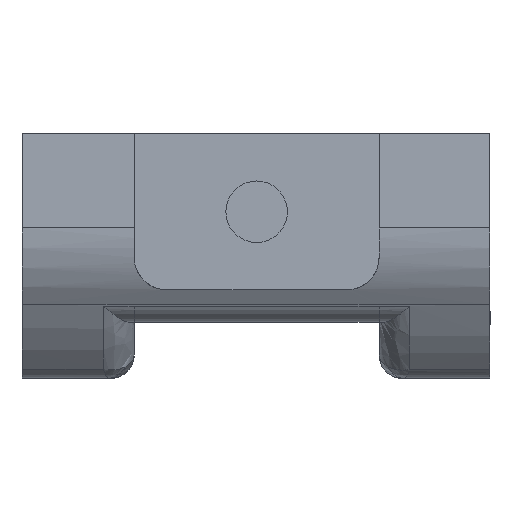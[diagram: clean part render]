
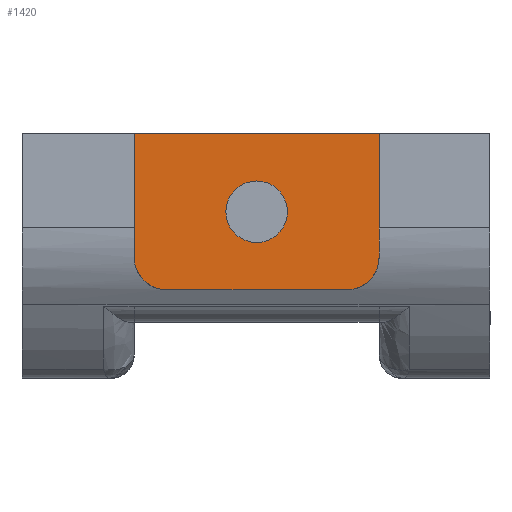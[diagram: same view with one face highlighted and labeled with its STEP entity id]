
A CAD part, front view. The second image highlights one B-rep face of the part: STEP entity #1420.
In plain terms, the highlighted planar face has unit normal (0, -1, 0).
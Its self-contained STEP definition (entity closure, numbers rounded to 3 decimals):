
#122 = AXIS2_PLACEMENT_3D ( 'NONE', #3254, #1624, #817 ) ;
#136 = VERTEX_POINT ( 'NONE', #1175 ) ;
#145 = ORIENTED_EDGE ( 'NONE', *, *, #2261, .F. ) ;
#321 = EDGE_CURVE ( 'NONE', #1790, #3347, #2233, .T. ) ;
#439 = AXIS2_PLACEMENT_3D ( 'NONE', #2309, #3396, #2859 ) ;
#485 = CARTESIAN_POINT ( 'NONE',  ( 0., 3.175, -5.31 ) ) ;
#489 = EDGE_CURVE ( 'NONE', #3307, #1974, #1639, .T. ) ;
#499 = CIRCLE ( 'NONE', #439, 1.5 ) ;
#536 = CARTESIAN_POINT ( 'NONE',  ( -4.381, 3.175, -6.032 ) ) ;
#575 = ORIENTED_EDGE ( 'NONE', *, *, #489, .T. ) ;
#640 = LINE ( 'NONE', #1937, #2943 ) ;
#683 = FACE_BOUND ( 'NONE', #936, .T. ) ;
#817 = DIRECTION ( 'NONE',  ( 0., 0., -1. ) ) ;
#936 = EDGE_LOOP ( 'NONE', ( #2551, #145 ) ) ;
#1020 = CARTESIAN_POINT ( 'NONE',  ( 5.969, 3.175, 0. ) ) ;
#1175 = CARTESIAN_POINT ( 'NONE',  ( -5.969, 3.175, 0. ) ) ;
#1206 = CIRCLE ( 'NONE', #122, 1.5 ) ;
#1323 = VERTEX_POINT ( 'NONE', #3058 ) ;
#1327 = DIRECTION ( 'NONE',  ( 1., 0., 0. ) ) ;
#1420 = ADVANCED_FACE ( 'NONE', ( #683, #3159 ), #2079, .T. ) ;
#1427 = VECTOR ( 'NONE', #2597, 1000. ) ;
#1436 = VECTOR ( 'NONE', #2365, 1000. ) ;
#1464 = CARTESIAN_POINT ( 'NONE',  ( 4.381, 3.175, -6.032 ) ) ;
#1465 = AXIS2_PLACEMENT_3D ( 'NONE', #1464, #2593, #1481 ) ;
#1481 = DIRECTION ( 'NONE',  ( 0., 0., -1. ) ) ;
#1499 = LINE ( 'NONE', #2553, #1436 ) ;
#1611 = CARTESIAN_POINT ( 'NONE',  ( -5.969, 3.175, -6.032 ) ) ;
#1618 = ORIENTED_EDGE ( 'NONE', *, *, #2819, .T. ) ;
#1624 = DIRECTION ( 'NONE',  ( 0., -1., 0. ) ) ;
#1639 = CIRCLE ( 'NONE', #1465, 1.588 ) ;
#1778 = CARTESIAN_POINT ( 'NONE',  ( 0., 3.175, 0. ) ) ;
#1789 = CARTESIAN_POINT ( 'NONE',  ( 5.969, 3.175, 0. ) ) ;
#1790 = VERTEX_POINT ( 'NONE', #1611 ) ;
#1827 = EDGE_CURVE ( 'NONE', #3347, #3307, #2129, .T. ) ;
#1937 = CARTESIAN_POINT ( 'NONE',  ( 0., 3.175, 0. ) ) ;
#1974 = VERTEX_POINT ( 'NONE', #2014 ) ;
#1995 = EDGE_CURVE ( 'NONE', #2124, #1974, #3364, .T. ) ;
#2014 = CARTESIAN_POINT ( 'NONE',  ( 5.969, 3.175, -6.032 ) ) ;
#2059 = DIRECTION ( 'NONE',  ( 0., -1., 0. ) ) ;
#2062 = DIRECTION ( 'NONE',  ( 0., -1., 0. ) ) ;
#2079 = PLANE ( 'NONE',  #2148 ) ;
#2116 = DIRECTION ( 'NONE',  ( 0., 0., -1. ) ) ;
#2124 = VERTEX_POINT ( 'NONE', #1789 ) ;
#2129 = LINE ( 'NONE', #3514, #2329 ) ;
#2148 = AXIS2_PLACEMENT_3D ( 'NONE', #1778, #2062, #2116 ) ;
#2233 = CIRCLE ( 'NONE', #2650, 1.588 ) ;
#2261 = EDGE_CURVE ( 'NONE', #1323, #3066, #1206, .T. ) ;
#2309 = CARTESIAN_POINT ( 'NONE',  ( 0., 3.175, -3.81 ) ) ;
#2329 = VECTOR ( 'NONE', #1327, 1000. ) ;
#2365 = DIRECTION ( 'NONE',  ( 0., 0., -1. ) ) ;
#2409 = EDGE_CURVE ( 'NONE', #136, #1790, #1499, .T. ) ;
#2490 = EDGE_CURVE ( 'NONE', #3066, #1323, #499, .T. ) ;
#2551 = ORIENTED_EDGE ( 'NONE', *, *, #2490, .F. ) ;
#2553 = CARTESIAN_POINT ( 'NONE',  ( -5.969, 3.175, 0. ) ) ;
#2573 = CARTESIAN_POINT ( 'NONE',  ( 4.381, 3.175, -7.62 ) ) ;
#2593 = DIRECTION ( 'NONE',  ( 0., -1., 0. ) ) ;
#2597 = DIRECTION ( 'NONE',  ( 0., 0., -1. ) ) ;
#2650 = AXIS2_PLACEMENT_3D ( 'NONE', #536, #2059, #3158 ) ;
#2742 = ORIENTED_EDGE ( 'NONE', *, *, #321, .T. ) ;
#2819 = EDGE_CURVE ( 'NONE', #2124, #136, #640, .T. ) ;
#2859 = DIRECTION ( 'NONE',  ( 0., 0., -1. ) ) ;
#2943 = VECTOR ( 'NONE', #3021, 1000. ) ;
#3021 = DIRECTION ( 'NONE',  ( -1., 0., 0. ) ) ;
#3058 = CARTESIAN_POINT ( 'NONE',  ( 0., 3.175, -2.31 ) ) ;
#3066 = VERTEX_POINT ( 'NONE', #485 ) ;
#3158 = DIRECTION ( 'NONE',  ( 0., 0., -1. ) ) ;
#3159 = FACE_OUTER_BOUND ( 'NONE', #3174, .T. ) ;
#3174 = EDGE_LOOP ( 'NONE', ( #3218, #2742, #3224, #575, #3355, #1618 ) ) ;
#3218 = ORIENTED_EDGE ( 'NONE', *, *, #2409, .T. ) ;
#3224 = ORIENTED_EDGE ( 'NONE', *, *, #1827, .T. ) ;
#3254 = CARTESIAN_POINT ( 'NONE',  ( 0., 3.175, -3.81 ) ) ;
#3307 = VERTEX_POINT ( 'NONE', #2573 ) ;
#3347 = VERTEX_POINT ( 'NONE', #3489 ) ;
#3355 = ORIENTED_EDGE ( 'NONE', *, *, #1995, .F. ) ;
#3364 = LINE ( 'NONE', #1020, #1427 ) ;
#3396 = DIRECTION ( 'NONE',  ( 0., -1., 0. ) ) ;
#3489 = CARTESIAN_POINT ( 'NONE',  ( -4.381, 3.175, -7.62 ) ) ;
#3514 = CARTESIAN_POINT ( 'NONE',  ( 0., 3.175, -7.62 ) ) ;
